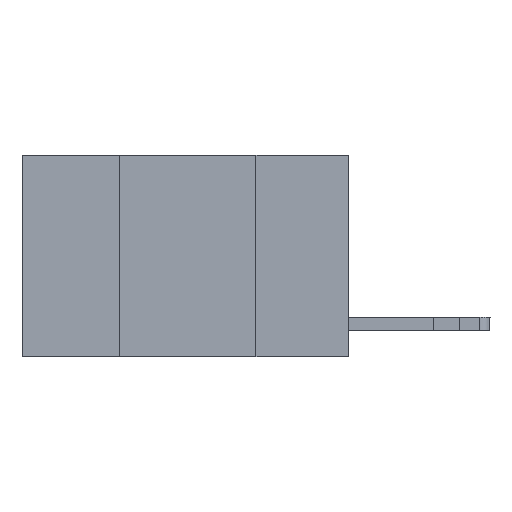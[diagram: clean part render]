
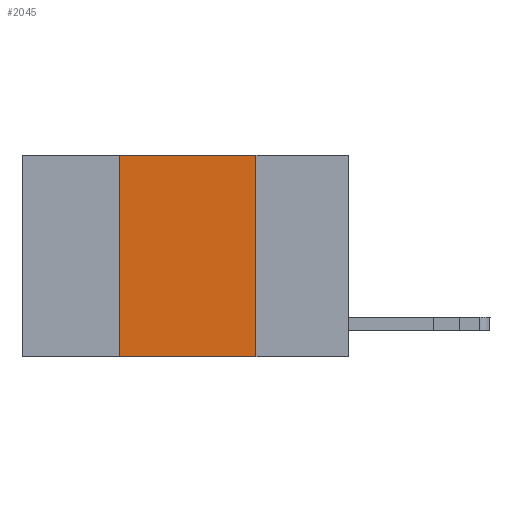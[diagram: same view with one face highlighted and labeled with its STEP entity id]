
A CAD part, left-side view. The second image highlights one B-rep face of the part: STEP entity #2045.
In plain terms, the highlighted planar face has unit normal (-1, 0, 0).
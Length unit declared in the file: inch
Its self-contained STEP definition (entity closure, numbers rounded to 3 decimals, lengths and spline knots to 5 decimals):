
#67 = VECTOR ( 'NONE', #16976, 39.37008 ) ;
#356 = PLANE ( 'NONE',  #5815 ) ;
#1190 = EDGE_CURVE ( 'NONE', #6687, #2074, #1259, .T. ) ;
#1259 = LINE ( 'NONE', #7367, #15502 ) ;
#1353 = VERTEX_POINT ( 'NONE', #7838 ) ;
#2045 = ADVANCED_FACE ( 'NONE', ( #4580 ), #356, .F. ) ;
#2074 = VERTEX_POINT ( 'NONE', #13418 ) ;
#2778 = CARTESIAN_POINT ( 'NONE',  ( 0., 0.42, 0. ) ) ;
#3140 = VECTOR ( 'NONE', #4205, 39.37008 ) ;
#3843 = VERTEX_POINT ( 'NONE', #14592 ) ;
#4205 = DIRECTION ( 'NONE',  ( 0., 0., 1. ) ) ;
#4343 = EDGE_CURVE ( 'NONE', #3843, #1353, #4748, .T. ) ;
#4580 = FACE_OUTER_BOUND ( 'NONE', #6097, .T. ) ;
#4748 = LINE ( 'NONE', #15572, #67 ) ;
#5815 = AXIS2_PLACEMENT_3D ( 'NONE', #9530, #9074, #6053 ) ;
#6053 = DIRECTION ( 'NONE',  ( 0., 0., -1. ) ) ;
#6097 = EDGE_LOOP ( 'NONE', ( #17125, #12181, #18283, #6496 ) ) ;
#6334 = LINE ( 'NONE', #9762, #17177 ) ;
#6496 = ORIENTED_EDGE ( 'NONE', *, *, #4343, .T. ) ;
#6687 = VERTEX_POINT ( 'NONE', #14687 ) ;
#7367 = CARTESIAN_POINT ( 'NONE',  ( 0., 0.6, 0. ) ) ;
#7838 = CARTESIAN_POINT ( 'NONE',  ( 0., 0.17, -0.37 ) ) ;
#9074 = DIRECTION ( 'NONE',  ( 1., 0., 0. ) ) ;
#9427 = DIRECTION ( 'NONE',  ( 0., -1., 0. ) ) ;
#9530 = CARTESIAN_POINT ( 'NONE',  ( 0., 0.6, 0. ) ) ;
#9762 = CARTESIAN_POINT ( 'NONE',  ( 0., 0.17, 0. ) ) ;
#12181 = ORIENTED_EDGE ( 'NONE', *, *, #1190, .F. ) ;
#13418 = CARTESIAN_POINT ( 'NONE',  ( 0., 0.17, 0. ) ) ;
#14020 = LINE ( 'NONE', #2778, #3140 ) ;
#14039 = DIRECTION ( 'NONE',  ( 0., 0., -1. ) ) ;
#14592 = CARTESIAN_POINT ( 'NONE',  ( 0., 0.42, -0.37 ) ) ;
#14687 = CARTESIAN_POINT ( 'NONE',  ( 0., 0.42, 0. ) ) ;
#15502 = VECTOR ( 'NONE', #9427, 39.37008 ) ;
#15549 = EDGE_CURVE ( 'NONE', #2074, #1353, #6334, .T. ) ;
#15572 = CARTESIAN_POINT ( 'NONE',  ( 0., 0.6, -0.37 ) ) ;
#16976 = DIRECTION ( 'NONE',  ( 0., -1., 0. ) ) ;
#17125 = ORIENTED_EDGE ( 'NONE', *, *, #15549, .F. ) ;
#17177 = VECTOR ( 'NONE', #14039, 39.37008 ) ;
#18094 = EDGE_CURVE ( 'NONE', #3843, #6687, #14020, .T. ) ;
#18283 = ORIENTED_EDGE ( 'NONE', *, *, #18094, .F. ) ;
